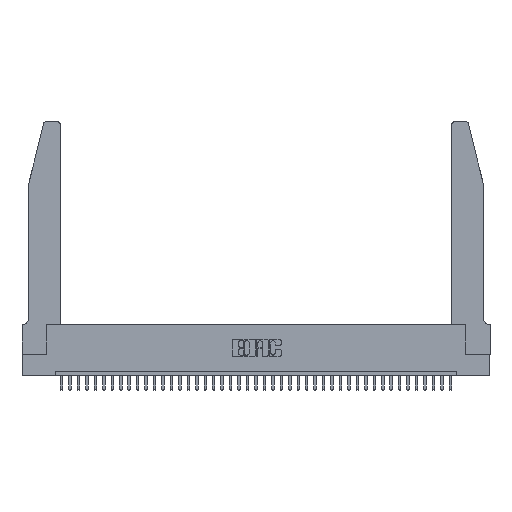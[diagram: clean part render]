
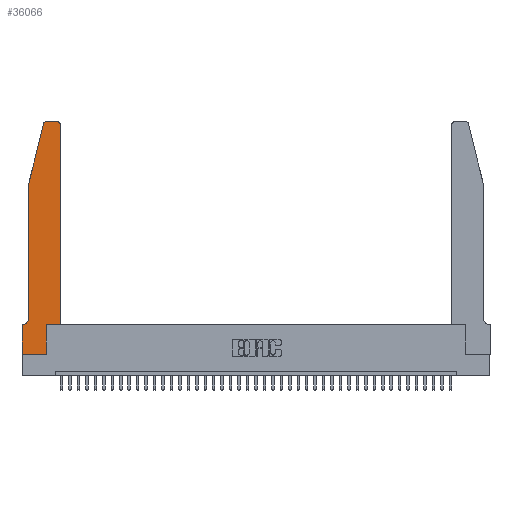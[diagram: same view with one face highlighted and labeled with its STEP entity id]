
A CAD part, top view. The second image highlights one B-rep face of the part: STEP entity #36066.
In plain terms, the highlighted planar face has unit normal (0, 0, 1).
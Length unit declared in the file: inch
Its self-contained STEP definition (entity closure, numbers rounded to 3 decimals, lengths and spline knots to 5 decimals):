
#746 = CARTESIAN_POINT ( 'NONE',  ( 0.2865, 0.35, 0.37 ) ) ;
#774 = ORIENTED_EDGE ( 'NONE', *, *, #32160, .T. ) ;
#999 = ORIENTED_EDGE ( 'NONE', *, *, #4201, .T. ) ;
#1283 = CARTESIAN_POINT ( 'NONE',  ( 0.4505, 2.72, 0.37 ) ) ;
#2081 = DIRECTION ( 'NONE',  ( -1., 0., 0. ) ) ;
#2384 = ORIENTED_EDGE ( 'NONE', *, *, #34277, .T. ) ;
#2844 = VECTOR ( 'NONE', #2081, 39.37008 ) ;
#3882 = VERTEX_POINT ( 'NONE', #7899 ) ;
#4201 = EDGE_CURVE ( 'NONE', #7682, #9224, #31745, .T. ) ;
#4227 = FACE_OUTER_BOUND ( 'NONE', #11827, .T. ) ;
#4457 = CARTESIAN_POINT ( 'NONE',  ( 0.4505, 0.35, 0.37 ) ) ;
#4779 = LINE ( 'NONE', #746, #7112 ) ;
#5737 = CARTESIAN_POINT ( 'NONE',  ( 0.4205, 2.72, 0.37 ) ) ;
#5761 = VERTEX_POINT ( 'NONE', #9232 ) ;
#6470 = CARTESIAN_POINT ( 'NONE',  ( 0., 0.35, 0.37 ) ) ;
#7048 = CARTESIAN_POINT ( 'NONE',  ( 0.2865, 0.35, 0.37 ) ) ;
#7112 = VECTOR ( 'NONE', #13631, 39.37008 ) ;
#7682 = VERTEX_POINT ( 'NONE', #16930 ) ;
#7788 = DIRECTION ( 'NONE',  ( 1., 0., 0. ) ) ;
#7899 = CARTESIAN_POINT ( 'NONE',  ( 0.0755, 0.42, 0.37 ) ) ;
#8203 = VERTEX_POINT ( 'NONE', #13146 ) ;
#8218 = VECTOR ( 'NONE', #28026, 39.37008 ) ;
#8671 = ORIENTED_EDGE ( 'NONE', *, *, #35739, .T. ) ;
#9008 = DIRECTION ( 'NONE',  ( 0., 0., -1. ) ) ;
#9063 = LINE ( 'NONE', #34628, #38227 ) ;
#9224 = VERTEX_POINT ( 'NONE', #26731 ) ;
#9232 = CARTESIAN_POINT ( 'NONE',  ( 0., 0.35, 0.37 ) ) ;
#9297 = CARTESIAN_POINT ( 'NONE',  ( 0.0755, 2., 0.37 ) ) ;
#9462 = ORIENTED_EDGE ( 'NONE', *, *, #31321, .T. ) ;
#9482 = DIRECTION ( 'NONE',  ( 1., 0., 0. ) ) ;
#9541 = VERTEX_POINT ( 'NONE', #7048 ) ;
#9760 = VECTOR ( 'NONE', #16640, 39.37008 ) ;
#9762 = AXIS2_PLACEMENT_3D ( 'NONE', #14185, #29442, #7788 ) ;
#9871 = ORIENTED_EDGE ( 'NONE', *, *, #37728, .T. ) ;
#9935 = AXIS2_PLACEMENT_3D ( 'NONE', #6470, #30747, #9482 ) ;
#11140 = CARTESIAN_POINT ( 'NONE',  ( 0.0755, 0.35, 0.37 ) ) ;
#11145 = VERTEX_POINT ( 'NONE', #28185 ) ;
#11473 = ORIENTED_EDGE ( 'NONE', *, *, #25510, .T. ) ;
#11827 = EDGE_LOOP ( 'NONE', ( #2384, #774, #999, #27338, #9462, #8671, #23302, #11473, #29534, #18049, #9871, #39388 ) ) ;
#11978 = DIRECTION ( 'NONE',  ( 1., 0., 0. ) ) ;
#13061 = VERTEX_POINT ( 'NONE', #1283 ) ;
#13077 = EDGE_CURVE ( 'NONE', #5761, #8203, #29404, .T. ) ;
#13146 = CARTESIAN_POINT ( 'NONE',  ( 0., 0., 0.37 ) ) ;
#13324 = LINE ( 'NONE', #11140, #2844 ) ;
#13441 = LINE ( 'NONE', #21882, #8218 ) ;
#13467 = CARTESIAN_POINT ( 'NONE',  ( 0.0055, 0.35, 0.37 ) ) ;
#13631 = DIRECTION ( 'NONE',  ( 0., 1., 0. ) ) ;
#13872 = VERTEX_POINT ( 'NONE', #31878 ) ;
#13999 = VERTEX_POINT ( 'NONE', #13467 ) ;
#14185 = CARTESIAN_POINT ( 'NONE',  ( 0.284, 2.72, 0.37 ) ) ;
#15596 = LINE ( 'NONE', #16662, #31914 ) ;
#15906 = AXIS2_PLACEMENT_3D ( 'NONE', #18096, #9008, #27704 ) ;
#16503 = CARTESIAN_POINT ( 'NONE',  ( 0., 0., 0.37 ) ) ;
#16640 = DIRECTION ( 'NONE',  ( 0., -1., 0. ) ) ;
#16662 = CARTESIAN_POINT ( 'NONE',  ( 0.0755, 2., 0.37 ) ) ;
#16840 = EDGE_CURVE ( 'NONE', #13872, #9541, #4779, .T. ) ;
#16930 = CARTESIAN_POINT ( 'NONE',  ( 0.25487, 2.72718, 0.37 ) ) ;
#17148 = CARTESIAN_POINT ( 'NONE',  ( 0., 0., 0.37 ) ) ;
#17426 = VECTOR ( 'NONE', #18534, 39.37008 ) ;
#17537 = CIRCLE ( 'NONE', #29190, 0.03 ) ;
#18049 = ORIENTED_EDGE ( 'NONE', *, *, #26640, .T. ) ;
#18096 = CARTESIAN_POINT ( 'NONE',  ( 0.0055, 0.42, 0.37 ) ) ;
#18534 = DIRECTION ( 'NONE',  ( -0.239, -0.971, 0. ) ) ;
#21882 = CARTESIAN_POINT ( 'NONE',  ( 0.2605, 2.75, 0.37 ) ) ;
#21974 = CARTESIAN_POINT ( 'NONE',  ( 0.284, 2.75, 0.37 ) ) ;
#23302 = ORIENTED_EDGE ( 'NONE', *, *, #13077, .T. ) ;
#24412 = DIRECTION ( 'NONE',  ( 1., 0., 0. ) ) ;
#24750 = PLANE ( 'NONE',  #9935 ) ;
#25112 = VECTOR ( 'NONE', #28899, 39.37008 ) ;
#25510 = EDGE_CURVE ( 'NONE', #8203, #13872, #26442, .T. ) ;
#26275 = VERTEX_POINT ( 'NONE', #21974 ) ;
#26442 = LINE ( 'NONE', #17148, #35529 ) ;
#26640 = EDGE_CURVE ( 'NONE', #9541, #11145, #9063, .T. ) ;
#26731 = CARTESIAN_POINT ( 'NONE',  ( 0.0755, 2., 0.37 ) ) ;
#27338 = ORIENTED_EDGE ( 'NONE', *, *, #36796, .T. ) ;
#27704 = DIRECTION ( 'NONE',  ( -1., 0., 0. ) ) ;
#28026 = DIRECTION ( 'NONE',  ( -1., 0., 0. ) ) ;
#28185 = CARTESIAN_POINT ( 'NONE',  ( 0.4505, 0.35, 0.37 ) ) ;
#28478 = DIRECTION ( 'NONE',  ( 1., 0., 0. ) ) ;
#28899 = DIRECTION ( 'NONE',  ( 0., 1., 0. ) ) ;
#29098 = VERTEX_POINT ( 'NONE', #29500 ) ;
#29190 = AXIS2_PLACEMENT_3D ( 'NONE', #5737, #30049, #11978 ) ;
#29404 = LINE ( 'NONE', #16503, #9760 ) ;
#29442 = DIRECTION ( 'NONE',  ( 0., 0., 1. ) ) ;
#29500 = CARTESIAN_POINT ( 'NONE',  ( 0.4205, 2.75, 0.37 ) ) ;
#29534 = ORIENTED_EDGE ( 'NONE', *, *, #16840, .T. ) ;
#30049 = DIRECTION ( 'NONE',  ( 0., 0., 1. ) ) ;
#30747 = DIRECTION ( 'NONE',  ( 0., 0., 1. ) ) ;
#31321 = EDGE_CURVE ( 'NONE', #3882, #13999, #35235, .T. ) ;
#31745 = LINE ( 'NONE', #9297, #17426 ) ;
#31878 = CARTESIAN_POINT ( 'NONE',  ( 0.2865, 0., 0.37 ) ) ;
#31914 = VECTOR ( 'NONE', #32203, 39.37008 ) ;
#32160 = EDGE_CURVE ( 'NONE', #26275, #7682, #35511, .T. ) ;
#32203 = DIRECTION ( 'NONE',  ( 0., -1., 0. ) ) ;
#34277 = EDGE_CURVE ( 'NONE', #29098, #26275, #13441, .T. ) ;
#34628 = CARTESIAN_POINT ( 'NONE',  ( 0.4505, 0.35, 0.37 ) ) ;
#35235 = CIRCLE ( 'NONE', #15906, 0.07 ) ;
#35511 = CIRCLE ( 'NONE', #9762, 0.03 ) ;
#35529 = VECTOR ( 'NONE', #24412, 39.37008 ) ;
#35739 = EDGE_CURVE ( 'NONE', #13999, #5761, #13324, .T. ) ;
#36066 = ADVANCED_FACE ( 'NONE', ( #4227 ), #24750, .T. ) ;
#36796 = EDGE_CURVE ( 'NONE', #9224, #3882, #15596, .T. ) ;
#36961 = EDGE_CURVE ( 'NONE', #13061, #29098, #17537, .T. ) ;
#37728 = EDGE_CURVE ( 'NONE', #11145, #13061, #38522, .T. ) ;
#38227 = VECTOR ( 'NONE', #28478, 39.37008 ) ;
#38522 = LINE ( 'NONE', #4457, #25112 ) ;
#39388 = ORIENTED_EDGE ( 'NONE', *, *, #36961, .T. ) ;
